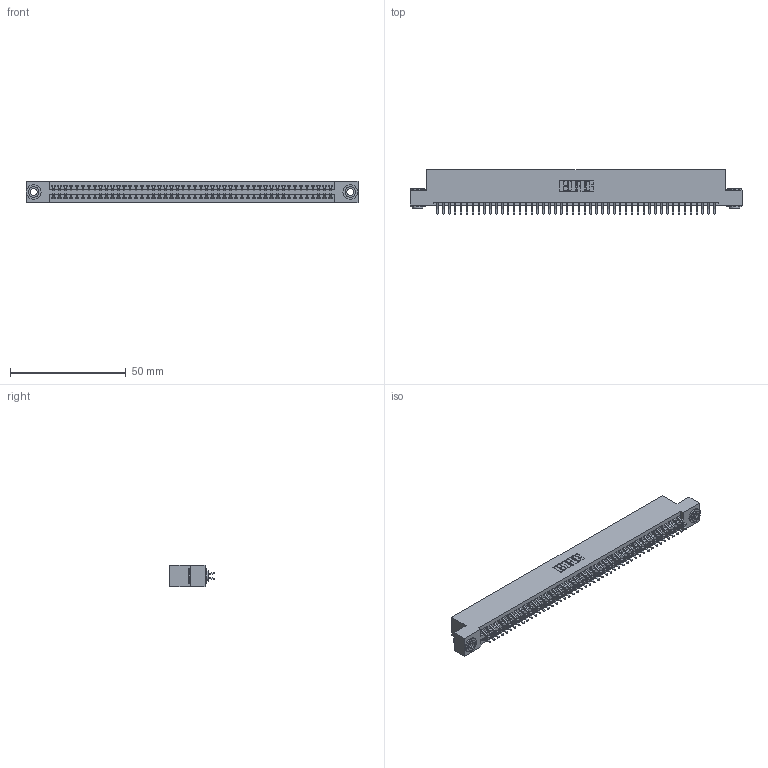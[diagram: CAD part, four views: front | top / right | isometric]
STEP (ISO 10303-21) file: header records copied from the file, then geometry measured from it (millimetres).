
FILE_DESCRIPTION (( 'STEP AP203' ), '1' );
FILE_NAME ('395-096-556-203.STEP', '2018-11-29T16:48:47', ( '' ), ( '' ), 'SwSTEP 2.0', 'SolidWorks 2016', '' );
FILE_SCHEMA (( 'CONFIG_CONTROL_DESIGN' ));
Length unit declared in the file: inch
Products named in the file (4): 345 Part_Flush Mounting Lugs - 0.156 Dia-TH; 395-096-556-203; 345-292-001_556 Tail; 345-250-002_345-250-002-102
Assembly tree (99 placements, depth 2):
  395-096-556-203
    345 Part_Flush Mounting Lugs - 0.156 Dia-TH
    345-292-001_556 Tail  x96
    345-250-002_345-250-002-102  x2
Bounding box: 143.13 x 19.24 x 9.4 mm (x, y, z)
Volume: 13975 mm3; surface area: 20894.4 mm2
Topology: 99 solids, 99 shells, 5540 faces, 16449 edges, 10834 vertices
Faces by surface type: plane 3642, cylinder 1890, cone 8
Entity records: 37724 total; most frequent: CARTESIAN_POINT 6307, ORIENTED_EDGE 6222, DIRECTION 5573, EDGE_CURVE 3111, VECTOR 2755, LINE 2755, VERTEX_POINT 2070, AXIS2_PLACEMENT_3D 1409
